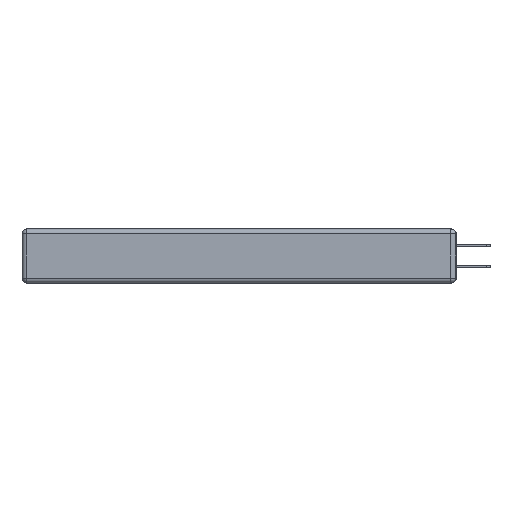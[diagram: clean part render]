
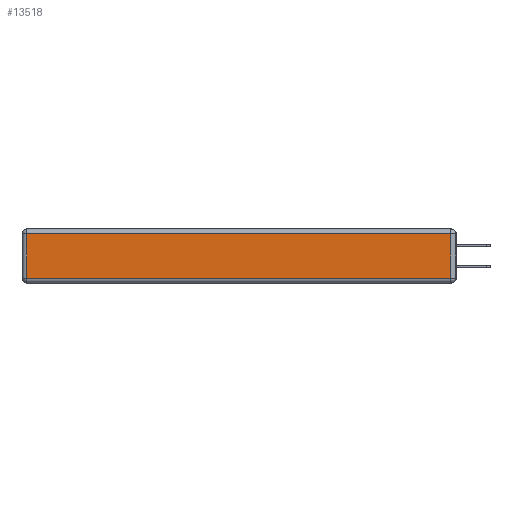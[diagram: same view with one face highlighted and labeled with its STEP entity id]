
A CAD part, left-side view. The second image highlights one B-rep face of the part: STEP entity #13518.
In plain terms, the highlighted planar face has unit normal (-1, 0, 0).
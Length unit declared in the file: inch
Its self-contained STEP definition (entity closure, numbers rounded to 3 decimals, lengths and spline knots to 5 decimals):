
#37 = EDGE_CURVE ( 'NONE', #15680, #20831, #11734, .T. ) ;
#1085 = CARTESIAN_POINT ( 'NONE',  ( 0., 0.03, -0.343 ) ) ;
#2395 = CARTESIAN_POINT ( 'NONE',  ( 0., 0.03, -0.313 ) ) ;
#3442 = VERTEX_POINT ( 'NONE', #2395 ) ;
#4309 = VECTOR ( 'NONE', #6564, 39.37008 ) ;
#4455 = VECTOR ( 'NONE', #12557, 39.37008 ) ;
#4461 = ORIENTED_EDGE ( 'NONE', *, *, #21148, .T. ) ;
#5586 = CARTESIAN_POINT ( 'NONE',  ( 0., 2.72, -0.343 ) ) ;
#5670 = AXIS2_PLACEMENT_3D ( 'NONE', #8753, #10397, #20251 ) ;
#6525 = DIRECTION ( 'NONE',  ( 0., -1., 0. ) ) ;
#6564 = DIRECTION ( 'NONE',  ( 0., 1., 0. ) ) ;
#7564 = ORIENTED_EDGE ( 'NONE', *, *, #37, .T. ) ;
#7922 = EDGE_CURVE ( 'NONE', #3442, #8209, #11635, .T. ) ;
#8209 = VERTEX_POINT ( 'NONE', #13271 ) ;
#8753 = CARTESIAN_POINT ( 'NONE',  ( 0., 0., -0.343 ) ) ;
#10045 = CARTESIAN_POINT ( 'NONE',  ( 0., 0., -0.313 ) ) ;
#10060 = ORIENTED_EDGE ( 'NONE', *, *, #7922, .T. ) ;
#10397 = DIRECTION ( 'NONE',  ( -1., 0., 0. ) ) ;
#10633 = CARTESIAN_POINT ( 'NONE',  ( 0., 2.72, -0.03 ) ) ;
#10676 = CARTESIAN_POINT ( 'NONE',  ( 0., 2.72, -0.313 ) ) ;
#11425 = FACE_OUTER_BOUND ( 'NONE', #16131, .T. ) ;
#11635 = LINE ( 'NONE', #1085, #4455 ) ;
#11734 = LINE ( 'NONE', #5586, #13292 ) ;
#12557 = DIRECTION ( 'NONE',  ( 0., 0., 1. ) ) ;
#12800 = ORIENTED_EDGE ( 'NONE', *, *, #15422, .T. ) ;
#13073 = VECTOR ( 'NONE', #6525, 39.37008 ) ;
#13271 = CARTESIAN_POINT ( 'NONE',  ( 0., 0.03, -0.03 ) ) ;
#13292 = VECTOR ( 'NONE', #16830, 39.37008 ) ;
#13518 = ADVANCED_FACE ( 'NONE', ( #11425 ), #20322, .T. ) ;
#14106 = LINE ( 'NONE', #10045, #13073 ) ;
#14778 = CARTESIAN_POINT ( 'NONE',  ( 0., 2.75, -0.03 ) ) ;
#15422 = EDGE_CURVE ( 'NONE', #20831, #3442, #14106, .T. ) ;
#15680 = VERTEX_POINT ( 'NONE', #10633 ) ;
#16131 = EDGE_LOOP ( 'NONE', ( #12800, #10060, #4461, #7564 ) ) ;
#16830 = DIRECTION ( 'NONE',  ( 0., 0., -1. ) ) ;
#19944 = LINE ( 'NONE', #14778, #4309 ) ;
#20251 = DIRECTION ( 'NONE',  ( 0., 0., 1. ) ) ;
#20322 = PLANE ( 'NONE',  #5670 ) ;
#20831 = VERTEX_POINT ( 'NONE', #10676 ) ;
#21148 = EDGE_CURVE ( 'NONE', #8209, #15680, #19944, .T. ) ;
